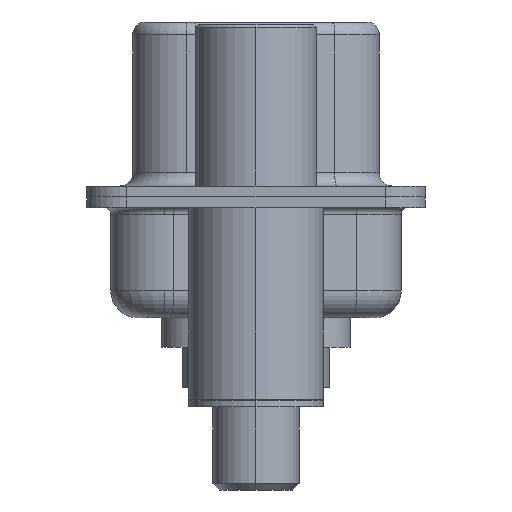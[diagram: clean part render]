
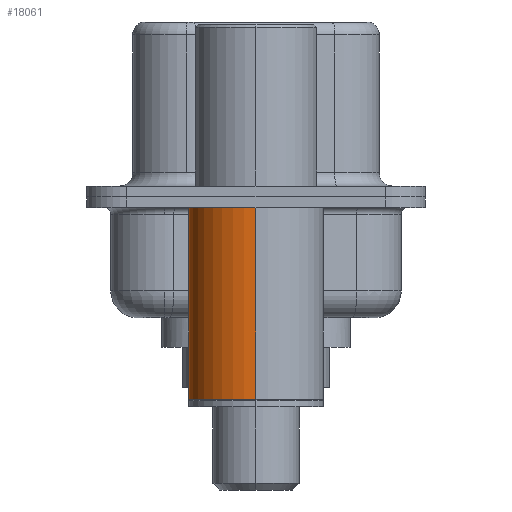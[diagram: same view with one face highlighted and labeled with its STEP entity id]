
A CAD part, left-side view. The second image highlights one B-rep face of the part: STEP entity #18061.
In plain terms, the highlighted cylindrical face has radius 2.5 mm (diameter 5 mm), a partial arc.
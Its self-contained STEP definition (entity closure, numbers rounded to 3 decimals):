
#1905 = DIRECTION ( 'NONE',  ( 1., 0., 0. ) ) ;
#1935 = DIRECTION ( 'NONE',  ( 0., 0., 1. ) ) ;
#1974 = CARTESIAN_POINT ( 'NONE',  ( 0., 0., -0.4 ) ) ;
#2412 = AXIS2_PLACEMENT_3D ( 'NONE', #1974, #1935, #1905 ) ;
#2832 = VERTEX_POINT ( 'NONE', #20875 ) ;
#4303 = AXIS2_PLACEMENT_3D ( 'NONE', #17194, #7261, #18839 ) ;
#4751 = CIRCLE ( 'NONE', #2412, 2.5 ) ;
#5090 = LINE ( 'NONE', #6495, #13875 ) ;
#6465 = CARTESIAN_POINT ( 'NONE',  ( 2.5, 0., -0.4 ) ) ;
#6495 = CARTESIAN_POINT ( 'NONE',  ( -2.5, 0., 0.581 ) ) ;
#6826 = DIRECTION ( 'NONE',  ( 0., 0., 1. ) ) ;
#6952 = AXIS2_PLACEMENT_3D ( 'NONE', #16764, #6826, #18410 ) ;
#7261 = DIRECTION ( 'NONE',  ( 0., 0., 1. ) ) ;
#8192 = VERTEX_POINT ( 'NONE', #19196 ) ;
#8351 = FACE_OUTER_BOUND ( 'NONE', #11152, .T. ) ;
#8651 = DIRECTION ( 'NONE',  ( 0., 0., 1. ) ) ;
#8855 = CARTESIAN_POINT ( 'NONE',  ( 2.5, 0., -7.525 ) ) ;
#9004 = CIRCLE ( 'NONE', #4303, 2.5 ) ;
#9283 = EDGE_CURVE ( 'NONE', #20864, #2832, #4751, .T. ) ;
#11152 = EDGE_LOOP ( 'NONE', ( #19844, #17098, #15152, #12271 ) ) ;
#11827 = EDGE_CURVE ( 'NONE', #20413, #8192, #9004, .T. ) ;
#11991 = CARTESIAN_POINT ( 'NONE',  ( 2.5, 0., 0.581 ) ) ;
#12271 = ORIENTED_EDGE ( 'NONE', *, *, #15178, .F. ) ;
#12818 = LINE ( 'NONE', #11991, #13887 ) ;
#13875 = VECTOR ( 'NONE', #16438, 1000. ) ;
#13887 = VECTOR ( 'NONE', #8651, 1000. ) ;
#15152 = ORIENTED_EDGE ( 'NONE', *, *, #9283, .F. ) ;
#15178 = EDGE_CURVE ( 'NONE', #20413, #20864, #12818, .T. ) ;
#16438 = DIRECTION ( 'NONE',  ( 0., 0., 1. ) ) ;
#16600 = EDGE_CURVE ( 'NONE', #8192, #2832, #5090, .T. ) ;
#16764 = CARTESIAN_POINT ( 'NONE',  ( 0., 0., 0.581 ) ) ;
#17098 = ORIENTED_EDGE ( 'NONE', *, *, #16600, .T. ) ;
#17194 = CARTESIAN_POINT ( 'NONE',  ( 0., 0., -7.525 ) ) ;
#18061 = ADVANCED_FACE ( 'NONE', ( #8351 ), #20519, .T. ) ;
#18410 = DIRECTION ( 'NONE',  ( 1., 0., 0. ) ) ;
#18839 = DIRECTION ( 'NONE',  ( 1., 0., 0. ) ) ;
#19196 = CARTESIAN_POINT ( 'NONE',  ( -2.5, 0., -7.525 ) ) ;
#19844 = ORIENTED_EDGE ( 'NONE', *, *, #11827, .T. ) ;
#20413 = VERTEX_POINT ( 'NONE', #8855 ) ;
#20519 = CYLINDRICAL_SURFACE ( 'NONE', #6952, 2.5 ) ;
#20864 = VERTEX_POINT ( 'NONE', #6465 ) ;
#20875 = CARTESIAN_POINT ( 'NONE',  ( -2.5, 0., -0.4 ) ) ;
